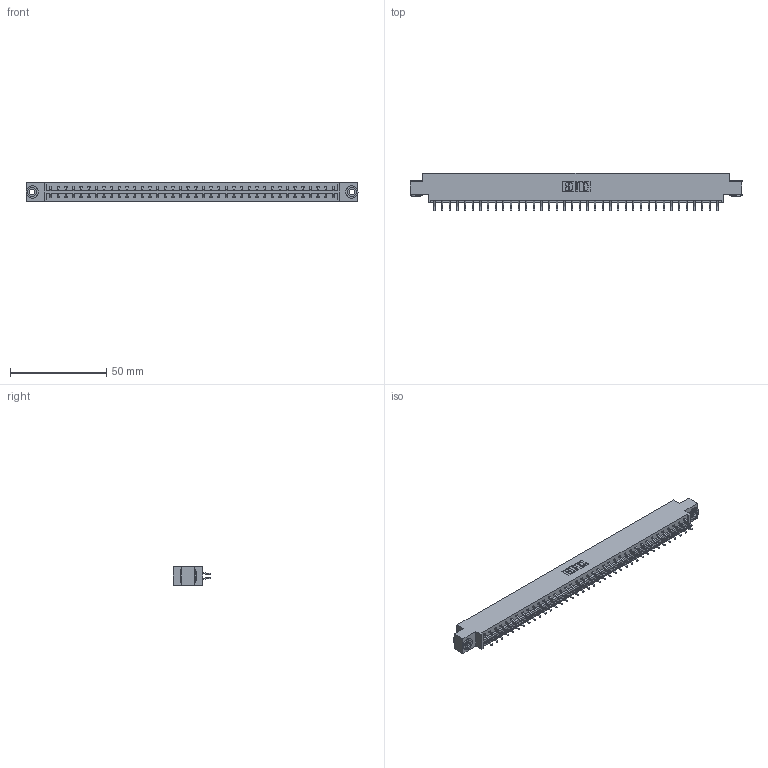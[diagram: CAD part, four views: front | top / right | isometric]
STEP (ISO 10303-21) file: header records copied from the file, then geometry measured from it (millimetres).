
FILE_DESCRIPTION (( 'STEP AP203' ), '1' );
FILE_NAME ('333-076-556-803.STEP', '2018-08-04T23:27:06', ( '' ), ( '' ), 'SwSTEP 2.0', 'SolidWorks 2016', '' );
FILE_SCHEMA (( 'CONFIG_CONTROL_DESIGN' ));
Length unit declared in the file: inch
Products named in the file (4): 333 Part_Offset - .156 Dia - TH; 345-292-001_556 Tail; 345-250-002_345-250-002-102; 333-076-556-803
Assembly tree (79 placements, depth 2):
  333-076-556-803
    333 Part_Offset - .156 Dia - TH
    345-292-001_556 Tail  x76
    345-250-002_345-250-002-102  x2
Bounding box: 172.11 x 19.57 x 9.4 mm (x, y, z)
Volume: 17322.7 mm3; surface area: 20803.5 mm2
Topology: 79 solids, 79 shells, 4564 faces, 13547 edges, 8926 vertices
Faces by surface type: plane 3124, cylinder 1432, cone 8
Entity records: 25966 total; most frequent: CARTESIAN_POINT 4301, ORIENTED_EDGE 4218, DIRECTION 3703, EDGE_CURVE 2109, LINE 1949, VECTOR 1949, VERTEX_POINT 1402, AXIS2_PLACEMENT_3D 877
